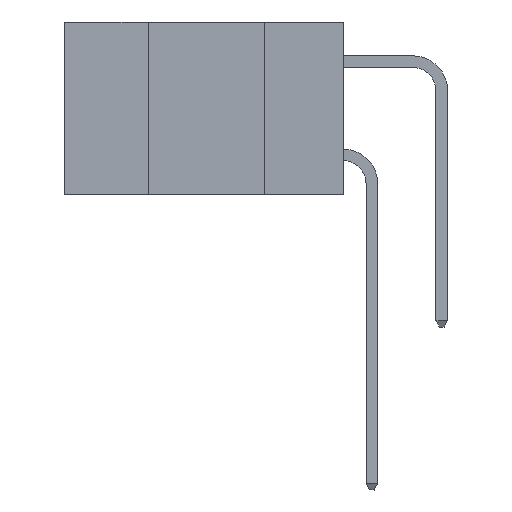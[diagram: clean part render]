
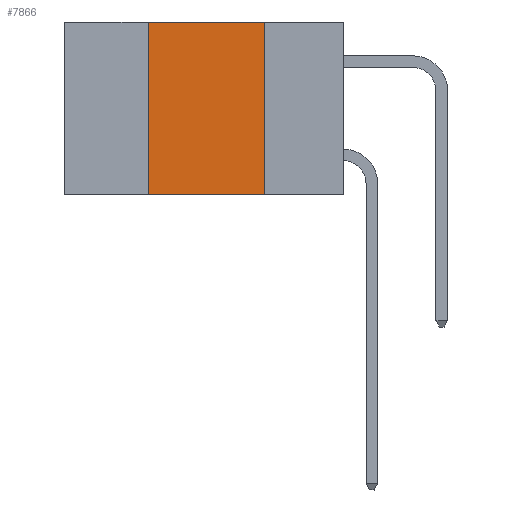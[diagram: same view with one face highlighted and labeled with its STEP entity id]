
A CAD part, left-side view. The second image highlights one B-rep face of the part: STEP entity #7866.
In plain terms, the highlighted planar face has unit normal (-1, 0, 0).
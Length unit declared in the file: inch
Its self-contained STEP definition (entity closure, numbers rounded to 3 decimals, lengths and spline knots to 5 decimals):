
#75 = CARTESIAN_POINT ( 'NONE',  ( 0., 0.42, -0.37 ) ) ;
#617 = CARTESIAN_POINT ( 'NONE',  ( 0., 0.42, -0.37 ) ) ;
#664 = CARTESIAN_POINT ( 'NONE',  ( 0., 0.6, 0. ) ) ;
#853 = VECTOR ( 'NONE', #1019, 39.37008 ) ;
#956 = LINE ( 'NONE', #75, #853 ) ;
#1019 = DIRECTION ( 'NONE',  ( 0., 0., 1. ) ) ;
#2451 = EDGE_CURVE ( 'NONE', #2978, #7271, #8214, .T. ) ;
#2648 = LINE ( 'NONE', #9503, #3545 ) ;
#2978 = VERTEX_POINT ( 'NONE', #5511 ) ;
#3431 = ORIENTED_EDGE ( 'NONE', *, *, #6336, .F. ) ;
#3456 = DIRECTION ( 'NONE',  ( 0., -1., 0. ) ) ;
#3545 = VECTOR ( 'NONE', #5747, 39.37008 ) ;
#4280 = CARTESIAN_POINT ( 'NONE',  ( 0., 0.17, -0.37 ) ) ;
#5102 = VERTEX_POINT ( 'NONE', #617 ) ;
#5119 = ORIENTED_EDGE ( 'NONE', *, *, #2451, .F. ) ;
#5511 = CARTESIAN_POINT ( 'NONE',  ( 0., 0.17, 0. ) ) ;
#5747 = DIRECTION ( 'NONE',  ( 0., -1., 0. ) ) ;
#6263 = VECTOR ( 'NONE', #3456, 39.37008 ) ;
#6336 = EDGE_CURVE ( 'NONE', #11952, #2978, #12002, .T. ) ;
#6487 = DIRECTION ( 'NONE',  ( 0., 0., -1. ) ) ;
#7271 = VERTEX_POINT ( 'NONE', #8233 ) ;
#7866 = ADVANCED_FACE ( 'NONE', ( #9129 ), #10211, .F. ) ;
#7925 = VECTOR ( 'NONE', #6487, 39.37008 ) ;
#8168 = EDGE_CURVE ( 'NONE', #5102, #11952, #956, .T. ) ;
#8188 = DIRECTION ( 'NONE',  ( 1., 0., 0. ) ) ;
#8214 = LINE ( 'NONE', #4280, #7925 ) ;
#8233 = CARTESIAN_POINT ( 'NONE',  ( 0., 0.17, -0.37 ) ) ;
#8592 = CARTESIAN_POINT ( 'NONE',  ( 0., 0.42, 0. ) ) ;
#8998 = DIRECTION ( 'NONE',  ( 0., 0., -1. ) ) ;
#9129 = FACE_OUTER_BOUND ( 'NONE', #9533, .T. ) ;
#9503 = CARTESIAN_POINT ( 'NONE',  ( 0., 0.6, -0.37 ) ) ;
#9533 = EDGE_LOOP ( 'NONE', ( #5119, #3431, #10738, #12337 ) ) ;
#10211 = PLANE ( 'NONE',  #12402 ) ;
#10738 = ORIENTED_EDGE ( 'NONE', *, *, #8168, .F. ) ;
#11847 = CARTESIAN_POINT ( 'NONE',  ( 0., 0.6, 0. ) ) ;
#11862 = EDGE_CURVE ( 'NONE', #5102, #7271, #2648, .T. ) ;
#11952 = VERTEX_POINT ( 'NONE', #8592 ) ;
#12002 = LINE ( 'NONE', #664, #6263 ) ;
#12337 = ORIENTED_EDGE ( 'NONE', *, *, #11862, .T. ) ;
#12402 = AXIS2_PLACEMENT_3D ( 'NONE', #11847, #8188, #8998 ) ;
